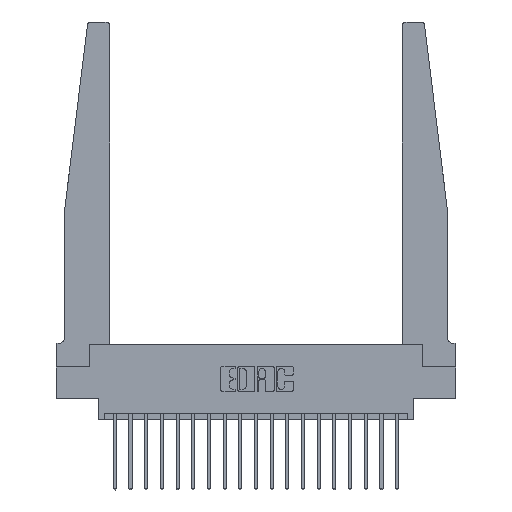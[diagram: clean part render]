
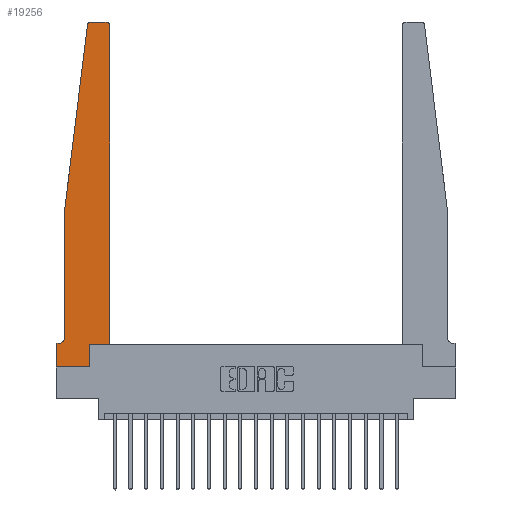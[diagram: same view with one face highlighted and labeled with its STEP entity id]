
A CAD part, top view. The second image highlights one B-rep face of the part: STEP entity #19256.
In plain terms, the highlighted planar face has unit normal (0, 0, 1).
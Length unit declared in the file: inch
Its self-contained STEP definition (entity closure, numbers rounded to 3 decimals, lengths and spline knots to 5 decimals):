
#9 = CIRCLE ( 'NONE', #3183, 0.03 ) ;
#25 = DIRECTION ( 'NONE',  ( 0., -1., 0. ) ) ;
#330 = CARTESIAN_POINT ( 'NONE',  ( 0.015, 0.1875, 0.37 ) ) ;
#497 = DIRECTION ( 'NONE',  ( 0., 0., -1. ) ) ;
#641 = CARTESIAN_POINT ( 'NONE',  ( 0.24675, 2.72367, 0.37 ) ) ;
#802 = VERTEX_POINT ( 'NONE', #641 ) ;
#816 = EDGE_CURVE ( 'NONE', #4122, #20164, #4694, .T. ) ;
#884 = AXIS2_PLACEMENT_3D ( 'NONE', #4328, #15381, #5958 ) ;
#907 = EDGE_CURVE ( 'NONE', #18037, #19869, #11652, .T. ) ;
#1008 = CARTESIAN_POINT ( 'NONE',  ( 0.27653, 2.75, 0.37 ) ) ;
#1018 = LINE ( 'NONE', #15816, #8937 ) ;
#1043 = DIRECTION ( 'NONE',  ( -0.122, -0.992, 0. ) ) ;
#1600 = ORIENTED_EDGE ( 'NONE', *, *, #14536, .T. ) ;
#1835 = DIRECTION ( 'NONE',  ( 0., 1., 0. ) ) ;
#1911 = DIRECTION ( 'NONE',  ( -1., 0., 0. ) ) ;
#1953 = FACE_OUTER_BOUND ( 'NONE', #14188, .T. ) ;
#1963 = AXIS2_PLACEMENT_3D ( 'NONE', #19372, #19446, #10022 ) ;
#2181 = LINE ( 'NONE', #8542, #10110 ) ;
#2247 = DIRECTION ( 'NONE',  ( -1., 0., 0. ) ) ;
#2621 = EDGE_CURVE ( 'NONE', #3224, #19936, #19990, .T. ) ;
#2629 = VECTOR ( 'NONE', #1043, 39.37008 ) ;
#3048 = CIRCLE ( 'NONE', #17200, 0.05 ) ;
#3065 = LINE ( 'NONE', #10472, #10999 ) ;
#3168 = DIRECTION ( 'NONE',  ( 0., 1., 0. ) ) ;
#3183 = AXIS2_PLACEMENT_3D ( 'NONE', #5104, #16161, #6700 ) ;
#3211 = VECTOR ( 'NONE', #17922, 39.37008 ) ;
#3224 = VERTEX_POINT ( 'NONE', #6447 ) ;
#3893 = VERTEX_POINT ( 'NONE', #18116 ) ;
#4122 = VERTEX_POINT ( 'NONE', #13947 ) ;
#4328 = CARTESIAN_POINT ( 'NONE',  ( 0.395, 2.72, 0.37 ) ) ;
#4694 = LINE ( 'NONE', #19228, #8949 ) ;
#5104 = CARTESIAN_POINT ( 'NONE',  ( 0.27653, 2.72, 0.37 ) ) ;
#5609 = ORIENTED_EDGE ( 'NONE', *, *, #16649, .T. ) ;
#5731 = CARTESIAN_POINT ( 'NONE',  ( 0.065, 1.25, 0.37 ) ) ;
#5958 = DIRECTION ( 'NONE',  ( 1., 0., 0. ) ) ;
#6447 = CARTESIAN_POINT ( 'NONE',  ( 0.425, 0.18, 0.37 ) ) ;
#6666 = CARTESIAN_POINT ( 'NONE',  ( 0.065, 0.2375, 0.37 ) ) ;
#6700 = DIRECTION ( 'NONE',  ( 1., 0., 0. ) ) ;
#7100 = EDGE_CURVE ( 'NONE', #20164, #802, #9, .T. ) ;
#7184 = ORIENTED_EDGE ( 'NONE', *, *, #9125, .T. ) ;
#7204 = ORIENTED_EDGE ( 'NONE', *, *, #20329, .T. ) ;
#7367 = ORIENTED_EDGE ( 'NONE', *, *, #10831, .T. ) ;
#7710 = CARTESIAN_POINT ( 'NONE',  ( 0., 0., 0.37 ) ) ;
#7972 = ORIENTED_EDGE ( 'NONE', *, *, #816, .T. ) ;
#8257 = ORIENTED_EDGE ( 'NONE', *, *, #18346, .T. ) ;
#8359 = ORIENTED_EDGE ( 'NONE', *, *, #10389, .T. ) ;
#8538 = VERTEX_POINT ( 'NONE', #19612 ) ;
#8542 = CARTESIAN_POINT ( 'NONE',  ( 0.065, 0.1875, 0.37 ) ) ;
#8768 = ORIENTED_EDGE ( 'NONE', *, *, #2621, .T. ) ;
#8937 = VECTOR ( 'NONE', #3168, 39.37008 ) ;
#8949 = VECTOR ( 'NONE', #1911, 39.37008 ) ;
#9125 = EDGE_CURVE ( 'NONE', #802, #18037, #11043, .T. ) ;
#9325 = VERTEX_POINT ( 'NONE', #17309 ) ;
#9972 = CARTESIAN_POINT ( 'NONE',  ( 0.015, 0.2375, 0.37 ) ) ;
#10001 = CARTESIAN_POINT ( 'NONE',  ( 0.425, 2.72, 0.37 ) ) ;
#10022 = DIRECTION ( 'NONE',  ( 1., 0., 0. ) ) ;
#10110 = VECTOR ( 'NONE', #2247, 39.37008 ) ;
#10259 = LINE ( 'NONE', #14149, #18626 ) ;
#10389 = EDGE_CURVE ( 'NONE', #3893, #3224, #3065, .T. ) ;
#10472 = CARTESIAN_POINT ( 'NONE',  ( 0.425, 0.18, 0.37 ) ) ;
#10625 = EDGE_CURVE ( 'NONE', #8538, #9325, #10259, .T. ) ;
#10831 = EDGE_CURVE ( 'NONE', #19869, #19838, #3048, .T. ) ;
#10999 = VECTOR ( 'NONE', #16870, 39.37008 ) ;
#11043 = LINE ( 'NONE', #5731, #2629 ) ;
#11554 = DIRECTION ( 'NONE',  ( -1., 0., 0. ) ) ;
#11615 = VECTOR ( 'NONE', #1835, 39.37008 ) ;
#11652 = LINE ( 'NONE', #17859, #3211 ) ;
#12838 = ORIENTED_EDGE ( 'NONE', *, *, #7100, .T. ) ;
#12876 = CARTESIAN_POINT ( 'NONE',  ( 0.065, 1.25, 0.37 ) ) ;
#12973 = ORIENTED_EDGE ( 'NONE', *, *, #907, .T. ) ;
#13308 = VERTEX_POINT ( 'NONE', #14976 ) ;
#13947 = CARTESIAN_POINT ( 'NONE',  ( 0.395, 2.75, 0.37 ) ) ;
#14017 = DIRECTION ( 'NONE',  ( 1., 0., 0. ) ) ;
#14149 = CARTESIAN_POINT ( 'NONE',  ( 0., 0., 0.37 ) ) ;
#14188 = EDGE_LOOP ( 'NONE', ( #7972, #12838, #7184, #12973, #7367, #1600, #17158, #7204, #8257, #8359, #8768, #5609 ) ) ;
#14536 = EDGE_CURVE ( 'NONE', #19838, #8538, #2181, .T. ) ;
#14976 = CARTESIAN_POINT ( 'NONE',  ( 0.2605, 0., 0.37 ) ) ;
#15381 = DIRECTION ( 'NONE',  ( 0., 0., 1. ) ) ;
#15514 = VECTOR ( 'NONE', #14017, 39.37008 ) ;
#15816 = CARTESIAN_POINT ( 'NONE',  ( 0.2605, 0.18, 0.37 ) ) ;
#15991 = CARTESIAN_POINT ( 'NONE',  ( 0.425, 0.18, 0.37 ) ) ;
#16028 = LINE ( 'NONE', #7710, #15514 ) ;
#16161 = DIRECTION ( 'NONE',  ( 0., 0., 1. ) ) ;
#16649 = EDGE_CURVE ( 'NONE', #19936, #4122, #16710, .T. ) ;
#16710 = CIRCLE ( 'NONE', #884, 0.03 ) ;
#16870 = DIRECTION ( 'NONE',  ( 1., 0., 0. ) ) ;
#17158 = ORIENTED_EDGE ( 'NONE', *, *, #10625, .T. ) ;
#17200 = AXIS2_PLACEMENT_3D ( 'NONE', #9972, #497, #11554 ) ;
#17309 = CARTESIAN_POINT ( 'NONE',  ( 0., 0., 0.37 ) ) ;
#17859 = CARTESIAN_POINT ( 'NONE',  ( 0.065, 1.25, 0.37 ) ) ;
#17870 = PLANE ( 'NONE',  #1963 ) ;
#17922 = DIRECTION ( 'NONE',  ( 0., -1., 0. ) ) ;
#18037 = VERTEX_POINT ( 'NONE', #12876 ) ;
#18116 = CARTESIAN_POINT ( 'NONE',  ( 0.2605, 0.18, 0.37 ) ) ;
#18346 = EDGE_CURVE ( 'NONE', #13308, #3893, #1018, .T. ) ;
#18626 = VECTOR ( 'NONE', #25, 39.37008 ) ;
#19228 = CARTESIAN_POINT ( 'NONE',  ( 0.25, 2.75, 0.37 ) ) ;
#19256 = ADVANCED_FACE ( 'NONE', ( #1953 ), #17870, .T. ) ;
#19372 = CARTESIAN_POINT ( 'NONE',  ( 0., 0.1875, 0.37 ) ) ;
#19446 = DIRECTION ( 'NONE',  ( 0., 0., 1. ) ) ;
#19612 = CARTESIAN_POINT ( 'NONE',  ( 0., 0.1875, 0.37 ) ) ;
#19838 = VERTEX_POINT ( 'NONE', #330 ) ;
#19869 = VERTEX_POINT ( 'NONE', #6666 ) ;
#19936 = VERTEX_POINT ( 'NONE', #10001 ) ;
#19990 = LINE ( 'NONE', #15991, #11615 ) ;
#20164 = VERTEX_POINT ( 'NONE', #1008 ) ;
#20329 = EDGE_CURVE ( 'NONE', #9325, #13308, #16028, .T. ) ;
